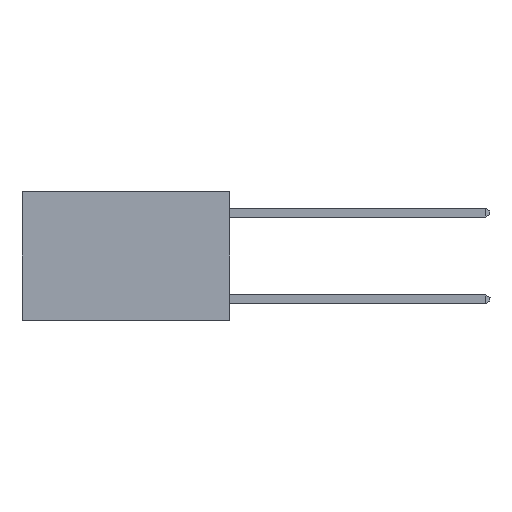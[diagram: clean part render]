
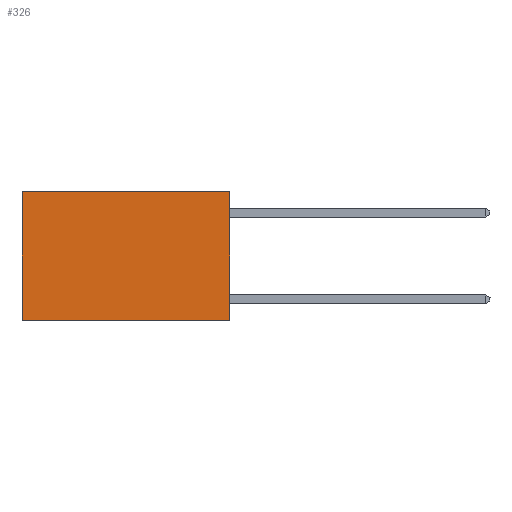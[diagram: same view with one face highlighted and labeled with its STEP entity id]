
A CAD part, left-side view. The second image highlights one B-rep face of the part: STEP entity #326.
In plain terms, the highlighted planar face has unit normal (-1, 0, 0).
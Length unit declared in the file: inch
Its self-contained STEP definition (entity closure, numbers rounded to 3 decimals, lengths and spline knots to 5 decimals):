
#286 = CARTESIAN_POINT ( 'NONE',  ( 0.2625, 0., 0. ) ) ;
#326 = ADVANCED_FACE ( 'NONE', ( #1816 ), #21894, .F. ) ;
#895 = AXIS2_PLACEMENT_3D ( 'NONE', #286, #11384, #7715 ) ;
#1816 = FACE_OUTER_BOUND ( 'NONE', #8729, .T. ) ;
#2209 = DIRECTION ( 'NONE',  ( 0., 0., -1. ) ) ;
#2596 = CARTESIAN_POINT ( 'NONE',  ( 0.2625, 0.6, 0. ) ) ;
#2733 = CARTESIAN_POINT ( 'NONE',  ( 0.2625, 0., -0.37 ) ) ;
#3433 = CARTESIAN_POINT ( 'NONE',  ( 0.2625, 0., 0. ) ) ;
#4208 = VERTEX_POINT ( 'NONE', #18507 ) ;
#4940 = VERTEX_POINT ( 'NONE', #2596 ) ;
#5223 = EDGE_CURVE ( 'NONE', #13934, #4208, #9328, .T. ) ;
#6406 = ORIENTED_EDGE ( 'NONE', *, *, #22696, .T. ) ;
#7086 = VECTOR ( 'NONE', #2209, 39.37008 ) ;
#7715 = DIRECTION ( 'NONE',  ( 0., 0., -1. ) ) ;
#8729 = EDGE_LOOP ( 'NONE', ( #6406, #21935, #23933, #15240 ) ) ;
#8786 = VECTOR ( 'NONE', #16835, 39.37008 ) ;
#9328 = LINE ( 'NONE', #11389, #8786 ) ;
#9672 = LINE ( 'NONE', #13795, #7086 ) ;
#10532 = DIRECTION ( 'NONE',  ( 0., 0., -1. ) ) ;
#10537 = LINE ( 'NONE', #21370, #11477 ) ;
#11384 = DIRECTION ( 'NONE',  ( 1., 0., 0. ) ) ;
#11389 = CARTESIAN_POINT ( 'NONE',  ( 0.2625, 0., -0.37 ) ) ;
#11477 = VECTOR ( 'NONE', #12378, 39.37008 ) ;
#12378 = DIRECTION ( 'NONE',  ( 0., 1., 0. ) ) ;
#12947 = LINE ( 'NONE', #20364, #16006 ) ;
#13795 = CARTESIAN_POINT ( 'NONE',  ( 0.2625, 0., 0. ) ) ;
#13934 = VERTEX_POINT ( 'NONE', #2733 ) ;
#14308 = EDGE_CURVE ( 'NONE', #15807, #4940, #10537, .T. ) ;
#15240 = ORIENTED_EDGE ( 'NONE', *, *, #14308, .T. ) ;
#15807 = VERTEX_POINT ( 'NONE', #3433 ) ;
#16006 = VECTOR ( 'NONE', #10532, 39.37008 ) ;
#16835 = DIRECTION ( 'NONE',  ( 0., 1., 0. ) ) ;
#18507 = CARTESIAN_POINT ( 'NONE',  ( 0.2625, 0.6, -0.37 ) ) ;
#20364 = CARTESIAN_POINT ( 'NONE',  ( 0.2625, 0.6, 0. ) ) ;
#21267 = EDGE_CURVE ( 'NONE', #15807, #13934, #9672, .T. ) ;
#21370 = CARTESIAN_POINT ( 'NONE',  ( 0.2625, 0., 0. ) ) ;
#21894 = PLANE ( 'NONE',  #895 ) ;
#21935 = ORIENTED_EDGE ( 'NONE', *, *, #5223, .F. ) ;
#22696 = EDGE_CURVE ( 'NONE', #4940, #4208, #12947, .T. ) ;
#23933 = ORIENTED_EDGE ( 'NONE', *, *, #21267, .F. ) ;
